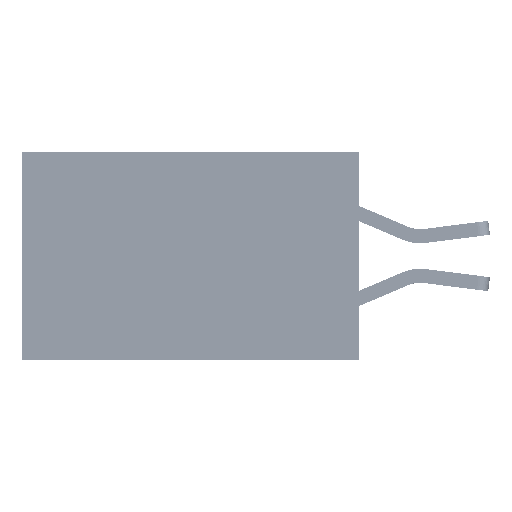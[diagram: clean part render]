
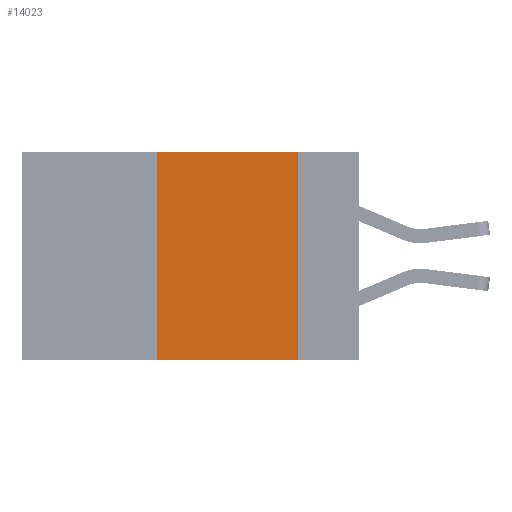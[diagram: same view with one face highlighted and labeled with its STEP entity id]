
A CAD part, left-side view. The second image highlights one B-rep face of the part: STEP entity #14023.
In plain terms, the highlighted planar face has unit normal (-1, 0, 0).
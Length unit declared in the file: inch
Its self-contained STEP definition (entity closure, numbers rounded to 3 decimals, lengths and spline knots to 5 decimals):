
#1376 = ORIENTED_EDGE ( 'NONE', *, *, #15603, .F. ) ;
#3969 = ORIENTED_EDGE ( 'NONE', *, *, #15575, .F. ) ;
#6026 = LINE ( 'NONE', #24953, #16531 ) ;
#6063 = DIRECTION ( 'NONE',  ( 1., 0., 0. ) ) ;
#7043 = VERTEX_POINT ( 'NONE', #23043 ) ;
#8426 = VECTOR ( 'NONE', #15376, 39.37008 ) ;
#8719 = DIRECTION ( 'NONE',  ( 0., 0., -1. ) ) ;
#9611 = VERTEX_POINT ( 'NONE', #34660 ) ;
#14023 = ADVANCED_FACE ( 'NONE', ( #22602 ), #37230, .F. ) ;
#15376 = DIRECTION ( 'NONE',  ( 0., 0., -1. ) ) ;
#15425 = VERTEX_POINT ( 'NONE', #27738 ) ;
#15575 = EDGE_CURVE ( 'NONE', #36337, #9611, #6026, .T. ) ;
#15603 = EDGE_CURVE ( 'NONE', #9611, #7043, #30455, .T. ) ;
#16531 = VECTOR ( 'NONE', #34100, 39.37008 ) ;
#18366 = EDGE_CURVE ( 'NONE', #36337, #15425, #21349, .T. ) ;
#20780 = EDGE_LOOP ( 'NONE', ( #39188, #1376, #3969, #38674 ) ) ;
#21349 = LINE ( 'NONE', #23514, #31745 ) ;
#22602 = FACE_OUTER_BOUND ( 'NONE', #20780, .T. ) ;
#22710 = CARTESIAN_POINT ( 'NONE',  ( 0., 0.6, 0. ) ) ;
#23043 = CARTESIAN_POINT ( 'NONE',  ( 0., 0.11, 0. ) ) ;
#23514 = CARTESIAN_POINT ( 'NONE',  ( 0., 0.6, -0.37 ) ) ;
#24953 = CARTESIAN_POINT ( 'NONE',  ( 0., 0.36, 0. ) ) ;
#26463 = VECTOR ( 'NONE', #38512, 39.37008 ) ;
#27738 = CARTESIAN_POINT ( 'NONE',  ( 0., 0.11, -0.37 ) ) ;
#30455 = LINE ( 'NONE', #22710, #26463 ) ;
#31745 = VECTOR ( 'NONE', #39582, 39.37008 ) ;
#34100 = DIRECTION ( 'NONE',  ( 0., 0., 1. ) ) ;
#34182 = EDGE_CURVE ( 'NONE', #7043, #15425, #40272, .T. ) ;
#34406 = CARTESIAN_POINT ( 'NONE',  ( 0., 0.11, 0. ) ) ;
#34660 = CARTESIAN_POINT ( 'NONE',  ( 0., 0.36, 0. ) ) ;
#36337 = VERTEX_POINT ( 'NONE', #38814 ) ;
#37230 = PLANE ( 'NONE',  #38430 ) ;
#38430 = AXIS2_PLACEMENT_3D ( 'NONE', #40707, #6063, #8719 ) ;
#38512 = DIRECTION ( 'NONE',  ( 0., -1., 0. ) ) ;
#38674 = ORIENTED_EDGE ( 'NONE', *, *, #18366, .T. ) ;
#38814 = CARTESIAN_POINT ( 'NONE',  ( 0., 0.36, -0.37 ) ) ;
#39188 = ORIENTED_EDGE ( 'NONE', *, *, #34182, .F. ) ;
#39582 = DIRECTION ( 'NONE',  ( 0., -1., 0. ) ) ;
#40272 = LINE ( 'NONE', #34406, #8426 ) ;
#40707 = CARTESIAN_POINT ( 'NONE',  ( 0., 0.6, 0. ) ) ;
